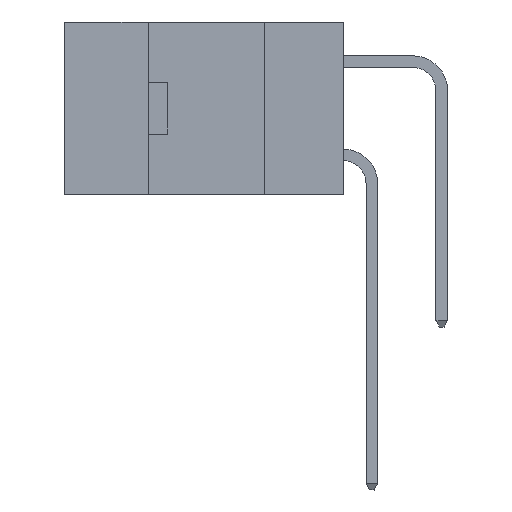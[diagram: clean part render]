
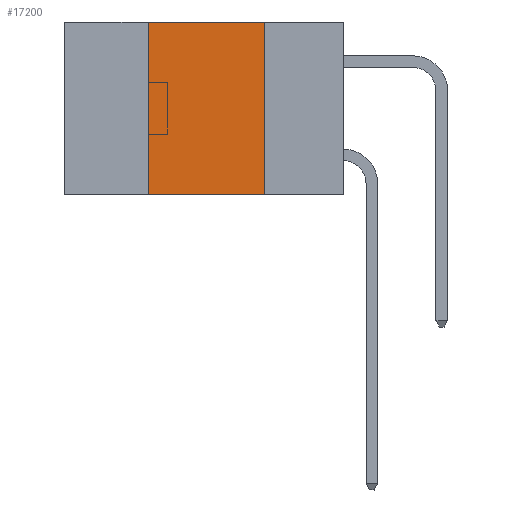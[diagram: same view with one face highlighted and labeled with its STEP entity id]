
A CAD part, left-side view. The second image highlights one B-rep face of the part: STEP entity #17200.
In plain terms, the highlighted planar face has unit normal (-1, 0, 0).
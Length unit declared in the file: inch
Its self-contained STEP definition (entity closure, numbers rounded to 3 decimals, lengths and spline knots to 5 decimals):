
#885 = CARTESIAN_POINT ( 'NONE',  ( 0., 0.42, -0.37 ) ) ;
#1622 = PLANE ( 'NONE',  #22436 ) ;
#1830 = VERTEX_POINT ( 'NONE', #29419 ) ;
#1976 = LINE ( 'NONE', #29920, #25292 ) ;
#2072 = CARTESIAN_POINT ( 'NONE',  ( 0., 0.6, 0. ) ) ;
#3291 = LINE ( 'NONE', #17067, #20033 ) ;
#4764 = LINE ( 'NONE', #28599, #7925 ) ;
#5233 = VECTOR ( 'NONE', #20152, 39.37008 ) ;
#6754 = ORIENTED_EDGE ( 'NONE', *, *, #28118, .F. ) ;
#7118 = EDGE_CURVE ( 'NONE', #24938, #21041, #4764, .T. ) ;
#7925 = VECTOR ( 'NONE', #23417, 39.37008 ) ;
#9242 = DIRECTION ( 'NONE',  ( 1., 0., 0. ) ) ;
#10319 = VERTEX_POINT ( 'NONE', #15827 ) ;
#12351 = ORIENTED_EDGE ( 'NONE', *, *, #13049, .F. ) ;
#13049 = EDGE_CURVE ( 'NONE', #10319, #21041, #27476, .T. ) ;
#15593 = ORIENTED_EDGE ( 'NONE', *, *, #18807, .F. ) ;
#15827 = CARTESIAN_POINT ( 'NONE',  ( 0., 0.17, 0. ) ) ;
#16800 = EDGE_LOOP ( 'NONE', ( #12351, #15593, #6754, #20587 ) ) ;
#17067 = CARTESIAN_POINT ( 'NONE',  ( 0., 0.6, 0. ) ) ;
#17200 = ADVANCED_FACE ( 'NONE', ( #22575 ), #1622, .F. ) ;
#18807 = EDGE_CURVE ( 'NONE', #1830, #10319, #3291, .T. ) ;
#20033 = VECTOR ( 'NONE', #26382, 39.37008 ) ;
#20152 = DIRECTION ( 'NONE',  ( 0., 0., -1. ) ) ;
#20587 = ORIENTED_EDGE ( 'NONE', *, *, #7118, .T. ) ;
#21041 = VERTEX_POINT ( 'NONE', #21601 ) ;
#21601 = CARTESIAN_POINT ( 'NONE',  ( 0., 0.17, -0.37 ) ) ;
#22436 = AXIS2_PLACEMENT_3D ( 'NONE', #2072, #9242, #29583 ) ;
#22575 = FACE_OUTER_BOUND ( 'NONE', #16800, .T. ) ;
#22914 = CARTESIAN_POINT ( 'NONE',  ( 0., 0.17, -0.37 ) ) ;
#23417 = DIRECTION ( 'NONE',  ( 0., -1., 0. ) ) ;
#24938 = VERTEX_POINT ( 'NONE', #885 ) ;
#25292 = VECTOR ( 'NONE', #25655, 39.37008 ) ;
#25655 = DIRECTION ( 'NONE',  ( 0., 0., 1. ) ) ;
#26382 = DIRECTION ( 'NONE',  ( 0., -1., 0. ) ) ;
#27476 = LINE ( 'NONE', #22914, #5233 ) ;
#28118 = EDGE_CURVE ( 'NONE', #24938, #1830, #1976, .T. ) ;
#28599 = CARTESIAN_POINT ( 'NONE',  ( 0., 0.6, -0.37 ) ) ;
#29419 = CARTESIAN_POINT ( 'NONE',  ( 0., 0.42, 0. ) ) ;
#29583 = DIRECTION ( 'NONE',  ( 0., 0., -1. ) ) ;
#29920 = CARTESIAN_POINT ( 'NONE',  ( 0., 0.42, -0.37 ) ) ;
